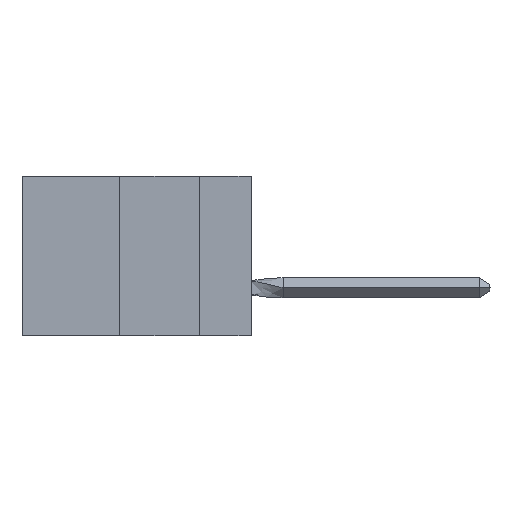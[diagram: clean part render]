
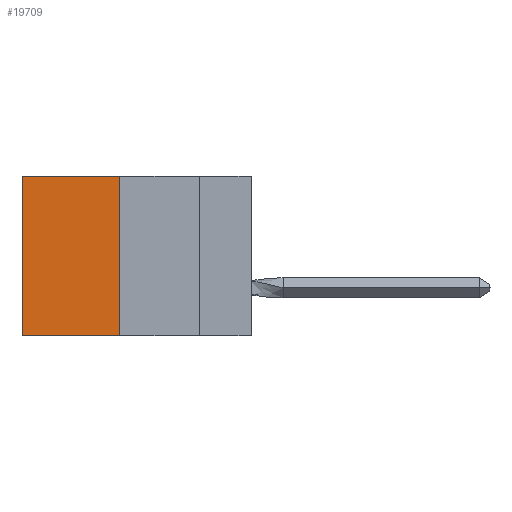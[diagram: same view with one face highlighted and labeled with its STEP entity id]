
A CAD part, left-side view. The second image highlights one B-rep face of the part: STEP entity #19709.
In plain terms, the highlighted planar face has unit normal (-1, 0, 0).
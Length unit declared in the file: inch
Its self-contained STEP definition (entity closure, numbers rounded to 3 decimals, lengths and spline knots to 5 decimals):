
#1462 = CARTESIAN_POINT ( 'NONE',  ( 0.305, 0.72, -0.5 ) ) ;
#2823 = VERTEX_POINT ( 'NONE', #15096 ) ;
#4467 = DIRECTION ( 'NONE',  ( 0., 0., -1. ) ) ;
#6104 = EDGE_CURVE ( 'NONE', #2823, #18884, #6400, .T. ) ;
#6400 = LINE ( 'NONE', #13600, #32473 ) ;
#7214 = ORIENTED_EDGE ( 'NONE', *, *, #9916, .F. ) ;
#7668 = LINE ( 'NONE', #1462, #26446 ) ;
#8940 = LINE ( 'NONE', #22545, #28567 ) ;
#9916 = EDGE_CURVE ( 'NONE', #18884, #35470, #8940, .T. ) ;
#10532 = VERTEX_POINT ( 'NONE', #25197 ) ;
#10969 = VECTOR ( 'NONE', #27447, 39.37008 ) ;
#11344 = ORIENTED_EDGE ( 'NONE', *, *, #20149, .T. ) ;
#11832 = ORIENTED_EDGE ( 'NONE', *, *, #25999, .T. ) ;
#13600 = CARTESIAN_POINT ( 'NONE',  ( 0.305, 0.413, -0.5 ) ) ;
#13663 = DIRECTION ( 'NONE',  ( 0., 0., -1. ) ) ;
#14414 = DIRECTION ( 'NONE',  ( 0., 1., 0. ) ) ;
#14538 = AXIS2_PLACEMENT_3D ( 'NONE', #22136, #16766, #13663 ) ;
#15096 = CARTESIAN_POINT ( 'NONE',  ( 0.305, 0.413, 0. ) ) ;
#16199 = FACE_OUTER_BOUND ( 'NONE', #20624, .T. ) ;
#16766 = DIRECTION ( 'NONE',  ( 1., 0., 0. ) ) ;
#17121 = CARTESIAN_POINT ( 'NONE',  ( 0.305, 0.72, -0.5 ) ) ;
#18884 = VERTEX_POINT ( 'NONE', #31653 ) ;
#19709 = ADVANCED_FACE ( 'NONE', ( #16199 ), #30394, .F. ) ;
#20149 = EDGE_CURVE ( 'NONE', #10532, #35470, #7668, .T. ) ;
#20624 = EDGE_LOOP ( 'NONE', ( #11344, #7214, #34819, #11832 ) ) ;
#22136 = CARTESIAN_POINT ( 'NONE',  ( 0.305, 0.413, -0.5 ) ) ;
#22545 = CARTESIAN_POINT ( 'NONE',  ( 0.305, 0.413, -0.5 ) ) ;
#25025 = CARTESIAN_POINT ( 'NONE',  ( 0.305, 0.413, 0. ) ) ;
#25197 = CARTESIAN_POINT ( 'NONE',  ( 0.305, 0.72, 0. ) ) ;
#25878 = LINE ( 'NONE', #25025, #10969 ) ;
#25999 = EDGE_CURVE ( 'NONE', #2823, #10532, #25878, .T. ) ;
#26446 = VECTOR ( 'NONE', #4467, 39.37008 ) ;
#27447 = DIRECTION ( 'NONE',  ( 0., 1., 0. ) ) ;
#27458 = DIRECTION ( 'NONE',  ( 0., 0., -1. ) ) ;
#28567 = VECTOR ( 'NONE', #14414, 39.37008 ) ;
#30394 = PLANE ( 'NONE',  #14538 ) ;
#31653 = CARTESIAN_POINT ( 'NONE',  ( 0.305, 0.413, -0.5 ) ) ;
#32473 = VECTOR ( 'NONE', #27458, 39.37008 ) ;
#34819 = ORIENTED_EDGE ( 'NONE', *, *, #6104, .F. ) ;
#35470 = VERTEX_POINT ( 'NONE', #17121 ) ;
